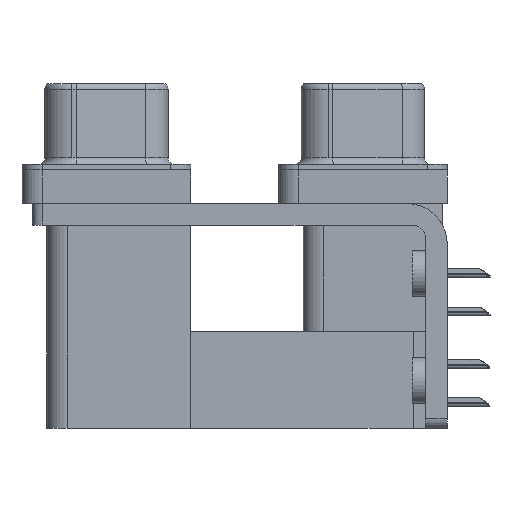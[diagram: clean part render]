
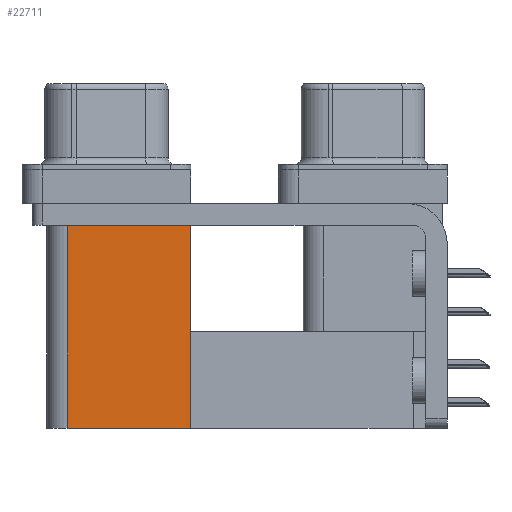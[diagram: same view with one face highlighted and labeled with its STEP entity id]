
A CAD part, left-side view. The second image highlights one B-rep face of the part: STEP entity #22711.
In plain terms, the highlighted planar face has unit normal (-1, 0, 0).
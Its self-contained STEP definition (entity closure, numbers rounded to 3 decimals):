
#29 = CARTESIAN_POINT ( 'NONE',  ( 3.7, 21.975, -19.2 ) ) ;
#717 = CARTESIAN_POINT ( 'NONE',  ( 3.7, 21.975, -19.2 ) ) ;
#1504 = DIRECTION ( 'NONE',  ( 0., 1., 0. ) ) ;
#2290 = VECTOR ( 'NONE', #7452, 1000. ) ;
#3207 = DIRECTION ( 'NONE',  ( 0., 1., 0. ) ) ;
#6557 = LINE ( 'NONE', #23601, #14198 ) ;
#7452 = DIRECTION ( 'NONE',  ( 0., 0., 1. ) ) ;
#7892 = VERTEX_POINT ( 'NONE', #39539 ) ;
#9057 = LINE ( 'NONE', #41918, #32710 ) ;
#12510 = DIRECTION ( 'NONE',  ( 0., 0., 1. ) ) ;
#14198 = VECTOR ( 'NONE', #19742, 1000. ) ;
#15709 = AXIS2_PLACEMENT_3D ( 'NONE', #18400, #40668, #1504 ) ;
#16569 = LINE ( 'NONE', #717, #2290 ) ;
#18400 = CARTESIAN_POINT ( 'NONE',  ( 3.7, 12.775, -19.2 ) ) ;
#19742 = DIRECTION ( 'NONE',  ( 0., 1., 0. ) ) ;
#20710 = EDGE_CURVE ( 'NONE', #40265, #27842, #16569, .T. ) ;
#21201 = EDGE_CURVE ( 'NONE', #7892, #27842, #6557, .T. ) ;
#21404 = FACE_OUTER_BOUND ( 'NONE', #41251, .T. ) ;
#22711 = ADVANCED_FACE ( 'NONE', ( #21404 ), #25085, .F. ) ;
#22912 = CARTESIAN_POINT ( 'NONE',  ( 3.7, 21.975, -2.5 ) ) ;
#22951 = CARTESIAN_POINT ( 'NONE',  ( 3.7, 12.775, -19.2 ) ) ;
#23047 = ORIENTED_EDGE ( 'NONE', *, *, #41078, .T. ) ;
#23601 = CARTESIAN_POINT ( 'NONE',  ( 3.7, 12.775, -2.5 ) ) ;
#25085 = PLANE ( 'NONE',  #15709 ) ;
#26404 = ORIENTED_EDGE ( 'NONE', *, *, #41219, .F. ) ;
#26538 = LINE ( 'NONE', #39739, #38910 ) ;
#27403 = ORIENTED_EDGE ( 'NONE', *, *, #21201, .T. ) ;
#27842 = VERTEX_POINT ( 'NONE', #22912 ) ;
#28148 = ORIENTED_EDGE ( 'NONE', *, *, #20710, .F. ) ;
#32710 = VECTOR ( 'NONE', #12510, 1000. ) ;
#36399 = VERTEX_POINT ( 'NONE', #22951 ) ;
#38910 = VECTOR ( 'NONE', #3207, 1000. ) ;
#39539 = CARTESIAN_POINT ( 'NONE',  ( 3.7, 12.775, -2.5 ) ) ;
#39739 = CARTESIAN_POINT ( 'NONE',  ( 3.7, 12.775, -19.2 ) ) ;
#40265 = VERTEX_POINT ( 'NONE', #29 ) ;
#40668 = DIRECTION ( 'NONE',  ( 1., 0., 0. ) ) ;
#41078 = EDGE_CURVE ( 'NONE', #36399, #7892, #9057, .T. ) ;
#41219 = EDGE_CURVE ( 'NONE', #36399, #40265, #26538, .T. ) ;
#41251 = EDGE_LOOP ( 'NONE', ( #27403, #28148, #26404, #23047 ) ) ;
#41918 = CARTESIAN_POINT ( 'NONE',  ( 3.7, 12.775, -19.2 ) ) ;
